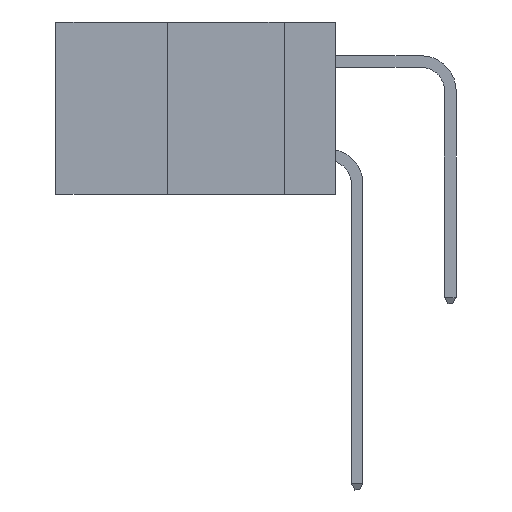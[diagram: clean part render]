
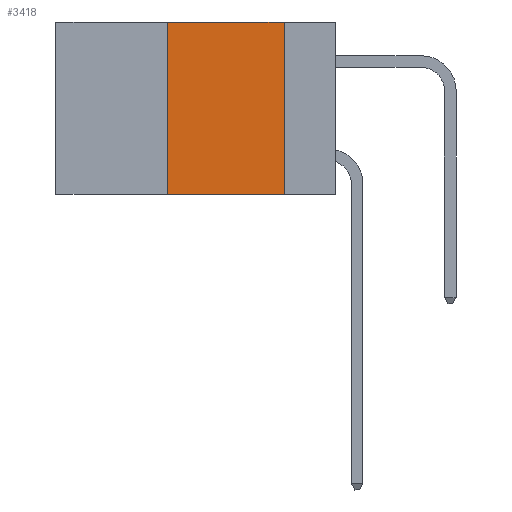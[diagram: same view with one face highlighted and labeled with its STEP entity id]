
A CAD part, left-side view. The second image highlights one B-rep face of the part: STEP entity #3418.
In plain terms, the highlighted planar face has unit normal (-1, 0, 0).
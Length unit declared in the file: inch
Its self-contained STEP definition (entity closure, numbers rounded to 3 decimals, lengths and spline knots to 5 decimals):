
#617 = EDGE_LOOP ( 'NONE', ( #15474, #10303, #20379, #18471 ) ) ;
#887 = LINE ( 'NONE', #1215, #4512 ) ;
#1215 = CARTESIAN_POINT ( 'NONE',  ( 0., 0.6, 0. ) ) ;
#1393 = EDGE_CURVE ( 'NONE', #6638, #6995, #17907, .T. ) ;
#1428 = DIRECTION ( 'NONE',  ( 1., 0., 0. ) ) ;
#2976 = CARTESIAN_POINT ( 'NONE',  ( 0., 0.36, 0. ) ) ;
#3302 = VERTEX_POINT ( 'NONE', #11161 ) ;
#3372 = CARTESIAN_POINT ( 'NONE',  ( 0., 0.36, -0.37 ) ) ;
#3418 = ADVANCED_FACE ( 'NONE', ( #19814 ), #16350, .F. ) ;
#3731 = CARTESIAN_POINT ( 'NONE',  ( 0., 0.11, 0. ) ) ;
#3831 = AXIS2_PLACEMENT_3D ( 'NONE', #16565, #1428, #14927 ) ;
#4225 = DIRECTION ( 'NONE',  ( 0., -1., 0. ) ) ;
#4512 = VECTOR ( 'NONE', #7881, 39.37008 ) ;
#6638 = VERTEX_POINT ( 'NONE', #3372 ) ;
#6995 = VERTEX_POINT ( 'NONE', #9819 ) ;
#7881 = DIRECTION ( 'NONE',  ( 0., -1., 0. ) ) ;
#9624 = VERTEX_POINT ( 'NONE', #11209 ) ;
#9819 = CARTESIAN_POINT ( 'NONE',  ( 0., 0.36, 0. ) ) ;
#10211 = VECTOR ( 'NONE', #4225, 39.37008 ) ;
#10303 = ORIENTED_EDGE ( 'NONE', *, *, #14190, .F. ) ;
#10939 = VECTOR ( 'NONE', #19639, 39.37008 ) ;
#11161 = CARTESIAN_POINT ( 'NONE',  ( 0., 0.11, -0.37 ) ) ;
#11209 = CARTESIAN_POINT ( 'NONE',  ( 0., 0.11, 0. ) ) ;
#14170 = CARTESIAN_POINT ( 'NONE',  ( 0., 0.6, -0.37 ) ) ;
#14190 = EDGE_CURVE ( 'NONE', #6995, #9624, #887, .T. ) ;
#14878 = EDGE_CURVE ( 'NONE', #9624, #3302, #20299, .T. ) ;
#14927 = DIRECTION ( 'NONE',  ( 0., 0., -1. ) ) ;
#15474 = ORIENTED_EDGE ( 'NONE', *, *, #14878, .F. ) ;
#15736 = DIRECTION ( 'NONE',  ( 0., 0., -1. ) ) ;
#16350 = PLANE ( 'NONE',  #3831 ) ;
#16565 = CARTESIAN_POINT ( 'NONE',  ( 0., 0.6, 0. ) ) ;
#17907 = LINE ( 'NONE', #2976, #10939 ) ;
#18471 = ORIENTED_EDGE ( 'NONE', *, *, #21201, .T. ) ;
#19141 = LINE ( 'NONE', #14170, #10211 ) ;
#19639 = DIRECTION ( 'NONE',  ( 0., 0., 1. ) ) ;
#19814 = FACE_OUTER_BOUND ( 'NONE', #617, .T. ) ;
#20299 = LINE ( 'NONE', #3731, #20865 ) ;
#20379 = ORIENTED_EDGE ( 'NONE', *, *, #1393, .F. ) ;
#20865 = VECTOR ( 'NONE', #15736, 39.37008 ) ;
#21201 = EDGE_CURVE ( 'NONE', #6638, #3302, #19141, .T. ) ;
